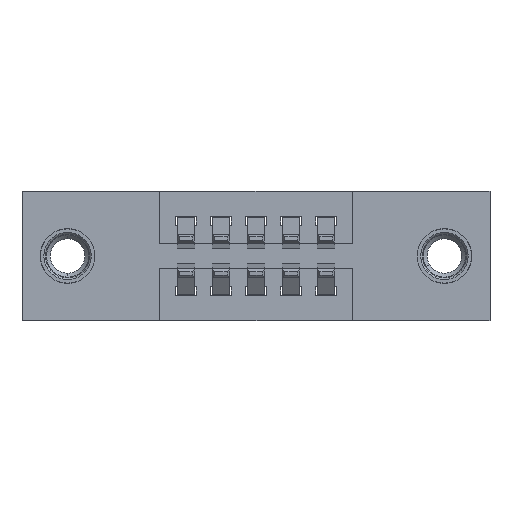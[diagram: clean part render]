
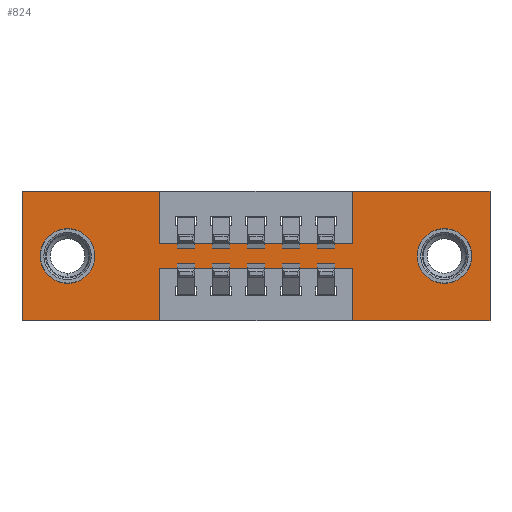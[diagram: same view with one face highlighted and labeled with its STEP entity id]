
A CAD part, front view. The second image highlights one B-rep face of the part: STEP entity #824.
In plain terms, the highlighted planar face has unit normal (0, -1, 0).
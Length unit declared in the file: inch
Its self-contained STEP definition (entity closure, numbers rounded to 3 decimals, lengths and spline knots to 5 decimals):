
#77 = CIRCLE ( 'NONE', #3202, 0.078 ) ;
#90 = EDGE_LOOP ( 'NONE', ( #3809, #7003 ) ) ;
#220 = DIRECTION ( 'NONE',  ( 0., 1., 0. ) ) ;
#221 = EDGE_CURVE ( 'NONE', #6655, #7467, #1801, .T. ) ;
#241 = ORIENTED_EDGE ( 'NONE', *, *, #6096, .T. ) ;
#418 = EDGE_CURVE ( 'NONE', #542, #6205, #9127, .T. ) ;
#452 = VECTOR ( 'NONE', #5190, 39.37008 ) ;
#530 = EDGE_CURVE ( 'NONE', #4119, #6771, #10148, .T. ) ;
#542 = VERTEX_POINT ( 'NONE', #4291 ) ;
#546 = DIRECTION ( 'NONE',  ( 0., 0., -1. ) ) ;
#575 = VECTOR ( 'NONE', #2495, 39.37008 ) ;
#582 = CARTESIAN_POINT ( 'NONE',  ( 0., 0., -0.37 ) ) ;
#590 = DIRECTION ( 'NONE',  ( -1., 0., 0. ) ) ;
#664 = CARTESIAN_POINT ( 'NONE',  ( 0., 0., 0. ) ) ;
#738 = CARTESIAN_POINT ( 'NONE',  ( 0.3925, 0., -0.37 ) ) ;
#788 = ORIENTED_EDGE ( 'NONE', *, *, #221, .F. ) ;
#824 = ADVANCED_FACE ( 'NONE', ( #9650, #1795, #8138 ), #9967, .T. ) ;
#829 = ORIENTED_EDGE ( 'NONE', *, *, #4914, .F. ) ;
#910 = CARTESIAN_POINT ( 'NONE',  ( 0.3925, 0., -0.15 ) ) ;
#934 = ORIENTED_EDGE ( 'NONE', *, *, #2771, .F. ) ;
#1058 = ORIENTED_EDGE ( 'NONE', *, *, #8251, .F. ) ;
#1175 = EDGE_CURVE ( 'NONE', #5970, #2832, #8995, .T. ) ;
#1290 = ORIENTED_EDGE ( 'NONE', *, *, #5078, .F. ) ;
#1302 = LINE ( 'NONE', #664, #9772 ) ;
#1352 = EDGE_CURVE ( 'NONE', #6100, #2262, #8988, .T. ) ;
#1418 = VERTEX_POINT ( 'NONE', #738 ) ;
#1430 = CARTESIAN_POINT ( 'NONE',  ( 1.335, 0., 0. ) ) ;
#1733 = DIRECTION ( 'NONE',  ( 0., 0., 1. ) ) ;
#1762 = VERTEX_POINT ( 'NONE', #7850 ) ;
#1776 = EDGE_CURVE ( 'NONE', #2832, #5970, #3116, .T. ) ;
#1795 = FACE_BOUND ( 'NONE', #8040, .T. ) ;
#1801 = LINE ( 'NONE', #4686, #7909 ) ;
#1920 = EDGE_LOOP ( 'NONE', ( #9890, #9005, #4966, #1058, #7486, #7089, #1290, #1922, #829, #788, #934, #9222 ) ) ;
#1922 = ORIENTED_EDGE ( 'NONE', *, *, #530, .F. ) ;
#2234 = EDGE_CURVE ( 'NONE', #8698, #1762, #7249, .T. ) ;
#2262 = VERTEX_POINT ( 'NONE', #6618 ) ;
#2304 = DIRECTION ( 'NONE',  ( 0., 0., -1. ) ) ;
#2336 = CARTESIAN_POINT ( 'NONE',  ( 0.3925, 0., 0. ) ) ;
#2426 = VERTEX_POINT ( 'NONE', #9957 ) ;
#2495 = DIRECTION ( 'NONE',  ( 0., 0., -1. ) ) ;
#2703 = CARTESIAN_POINT ( 'NONE',  ( 0.9425, 0., -0.37 ) ) ;
#2714 = CARTESIAN_POINT ( 'NONE',  ( 1.335, 0., 0. ) ) ;
#2771 = EDGE_CURVE ( 'NONE', #10098, #6655, #4522, .T. ) ;
#2789 = LINE ( 'NONE', #4511, #4870 ) ;
#2793 = AXIS2_PLACEMENT_3D ( 'NONE', #9621, #220, #1733 ) ;
#2832 = VERTEX_POINT ( 'NONE', #4194 ) ;
#2949 = CARTESIAN_POINT ( 'NONE',  ( 0.13, 0., -0.107 ) ) ;
#2990 = DIRECTION ( 'NONE',  ( 0., 1., 0. ) ) ;
#3001 = AXIS2_PLACEMENT_3D ( 'NONE', #4423, #2990, #3843 ) ;
#3116 = CIRCLE ( 'NONE', #5016, 0.078 ) ;
#3202 = AXIS2_PLACEMENT_3D ( 'NONE', #5303, #9335, #5408 ) ;
#3249 = VECTOR ( 'NONE', #5041, 39.37008 ) ;
#3771 = VECTOR ( 'NONE', #2304, 39.37008 ) ;
#3781 = DIRECTION ( 'NONE',  ( -1., 0., 0. ) ) ;
#3809 = ORIENTED_EDGE ( 'NONE', *, *, #1175, .T. ) ;
#3828 = DIRECTION ( 'NONE',  ( 1., 0., 0. ) ) ;
#3843 = DIRECTION ( 'NONE',  ( 0., 0., -1. ) ) ;
#4052 = CARTESIAN_POINT ( 'NONE',  ( 0.3925, 0., -0.15 ) ) ;
#4119 = VERTEX_POINT ( 'NONE', #910 ) ;
#4164 = DIRECTION ( 'NONE',  ( 0., 0., 1. ) ) ;
#4194 = CARTESIAN_POINT ( 'NONE',  ( 1.205, 0., -0.263 ) ) ;
#4269 = EDGE_CURVE ( 'NONE', #8076, #1418, #8939, .T. ) ;
#4291 = CARTESIAN_POINT ( 'NONE',  ( 0.13, 0., -0.263 ) ) ;
#4423 = CARTESIAN_POINT ( 'NONE',  ( 1.205, 0., -0.185 ) ) ;
#4436 = VECTOR ( 'NONE', #590, 39.37008 ) ;
#4511 = CARTESIAN_POINT ( 'NONE',  ( 0.9425, 0., 0. ) ) ;
#4516 = ORIENTED_EDGE ( 'NONE', *, *, #418, .T. ) ;
#4522 = LINE ( 'NONE', #6505, #8968 ) ;
#4561 = DIRECTION ( 'NONE',  ( 0., 0., -1. ) ) ;
#4642 = EDGE_CURVE ( 'NONE', #2262, #8076, #8435, .T. ) ;
#4664 = CARTESIAN_POINT ( 'NONE',  ( 0., 0., -0.37 ) ) ;
#4686 = CARTESIAN_POINT ( 'NONE',  ( 0., 0., 0. ) ) ;
#4870 = VECTOR ( 'NONE', #10045, 39.37008 ) ;
#4914 = EDGE_CURVE ( 'NONE', #7467, #4119, #5820, .T. ) ;
#4966 = ORIENTED_EDGE ( 'NONE', *, *, #1352, .F. ) ;
#5016 = AXIS2_PLACEMENT_3D ( 'NONE', #10058, #7691, #4561 ) ;
#5041 = DIRECTION ( 'NONE',  ( 0., 0., 1. ) ) ;
#5078 = EDGE_CURVE ( 'NONE', #6771, #2426, #2789, .T. ) ;
#5190 = DIRECTION ( 'NONE',  ( -1., 0., 0. ) ) ;
#5241 = DIRECTION ( 'NONE',  ( 0., -1., 0. ) ) ;
#5303 = CARTESIAN_POINT ( 'NONE',  ( 0.13, 0., -0.185 ) ) ;
#5408 = DIRECTION ( 'NONE',  ( 0., 0., 1. ) ) ;
#5820 = LINE ( 'NONE', #2336, #3771 ) ;
#5858 = CARTESIAN_POINT ( 'NONE',  ( 0.3925, 0., -0.22 ) ) ;
#5942 = CARTESIAN_POINT ( 'NONE',  ( 0., 0., -0.37 ) ) ;
#5970 = VERTEX_POINT ( 'NONE', #9173 ) ;
#6096 = EDGE_CURVE ( 'NONE', #6205, #542, #77, .T. ) ;
#6100 = VERTEX_POINT ( 'NONE', #9220 ) ;
#6205 = VERTEX_POINT ( 'NONE', #2949 ) ;
#6272 = LINE ( 'NONE', #5942, #4436 ) ;
#6425 = CARTESIAN_POINT ( 'NONE',  ( 0.3925, 0., -0.37 ) ) ;
#6450 = DIRECTION ( 'NONE',  ( 0., 0., -1. ) ) ;
#6505 = CARTESIAN_POINT ( 'NONE',  ( 0., 0., 0. ) ) ;
#6618 = CARTESIAN_POINT ( 'NONE',  ( 0.9425, 0., -0.22 ) ) ;
#6655 = VERTEX_POINT ( 'NONE', #8039 ) ;
#6771 = VERTEX_POINT ( 'NONE', #8496 ) ;
#6775 = EDGE_CURVE ( 'NONE', #2426, #8698, #1302, .T. ) ;
#6985 = CARTESIAN_POINT ( 'NONE',  ( 0.3925, 0., 0. ) ) ;
#7003 = ORIENTED_EDGE ( 'NONE', *, *, #1776, .T. ) ;
#7086 = DIRECTION ( 'NONE',  ( 1., 0., 0. ) ) ;
#7089 = ORIENTED_EDGE ( 'NONE', *, *, #6775, .F. ) ;
#7249 = LINE ( 'NONE', #2714, #7993 ) ;
#7297 = VECTOR ( 'NONE', #3781, 39.37008 ) ;
#7316 = EDGE_CURVE ( 'NONE', #1418, #10098, #9415, .T. ) ;
#7467 = VERTEX_POINT ( 'NONE', #6985 ) ;
#7486 = ORIENTED_EDGE ( 'NONE', *, *, #2234, .F. ) ;
#7569 = CARTESIAN_POINT ( 'NONE',  ( 0., 0., -0.37 ) ) ;
#7691 = DIRECTION ( 'NONE',  ( 0., 1., 0. ) ) ;
#7850 = CARTESIAN_POINT ( 'NONE',  ( 1.335, 0., -0.37 ) ) ;
#7909 = VECTOR ( 'NONE', #7086, 39.37008 ) ;
#7993 = VECTOR ( 'NONE', #6450, 39.37008 ) ;
#8029 = VECTOR ( 'NONE', #8078, 39.37008 ) ;
#8039 = CARTESIAN_POINT ( 'NONE',  ( 0., 0., 0. ) ) ;
#8040 = EDGE_LOOP ( 'NONE', ( #241, #4516 ) ) ;
#8076 = VERTEX_POINT ( 'NONE', #8930 ) ;
#8078 = DIRECTION ( 'NONE',  ( 1., 0., 0. ) ) ;
#8138 = FACE_OUTER_BOUND ( 'NONE', #1920, .T. ) ;
#8247 = AXIS2_PLACEMENT_3D ( 'NONE', #582, #5241, #546 ) ;
#8251 = EDGE_CURVE ( 'NONE', #1762, #6100, #6272, .T. ) ;
#8435 = LINE ( 'NONE', #5858, #452 ) ;
#8496 = CARTESIAN_POINT ( 'NONE',  ( 0.9425, 0., -0.15 ) ) ;
#8698 = VERTEX_POINT ( 'NONE', #1430 ) ;
#8930 = CARTESIAN_POINT ( 'NONE',  ( 0.3925, 0., -0.22 ) ) ;
#8939 = LINE ( 'NONE', #6425, #575 ) ;
#8968 = VECTOR ( 'NONE', #4164, 39.37008 ) ;
#8988 = LINE ( 'NONE', #2703, #3249 ) ;
#8995 = CIRCLE ( 'NONE', #3001, 0.078 ) ;
#9005 = ORIENTED_EDGE ( 'NONE', *, *, #4642, .F. ) ;
#9127 = CIRCLE ( 'NONE', #2793, 0.078 ) ;
#9173 = CARTESIAN_POINT ( 'NONE',  ( 1.205, 0., -0.107 ) ) ;
#9220 = CARTESIAN_POINT ( 'NONE',  ( 0.9425, 0., -0.37 ) ) ;
#9222 = ORIENTED_EDGE ( 'NONE', *, *, #7316, .F. ) ;
#9335 = DIRECTION ( 'NONE',  ( 0., 1., 0. ) ) ;
#9415 = LINE ( 'NONE', #7569, #7297 ) ;
#9621 = CARTESIAN_POINT ( 'NONE',  ( 0.13, 0., -0.185 ) ) ;
#9650 = FACE_BOUND ( 'NONE', #90, .T. ) ;
#9772 = VECTOR ( 'NONE', #3828, 39.37008 ) ;
#9890 = ORIENTED_EDGE ( 'NONE', *, *, #4269, .F. ) ;
#9957 = CARTESIAN_POINT ( 'NONE',  ( 0.9425, 0., 0. ) ) ;
#9967 = PLANE ( 'NONE',  #8247 ) ;
#10045 = DIRECTION ( 'NONE',  ( 0., 0., 1. ) ) ;
#10058 = CARTESIAN_POINT ( 'NONE',  ( 1.205, 0., -0.185 ) ) ;
#10098 = VERTEX_POINT ( 'NONE', #4664 ) ;
#10148 = LINE ( 'NONE', #4052, #8029 ) ;
